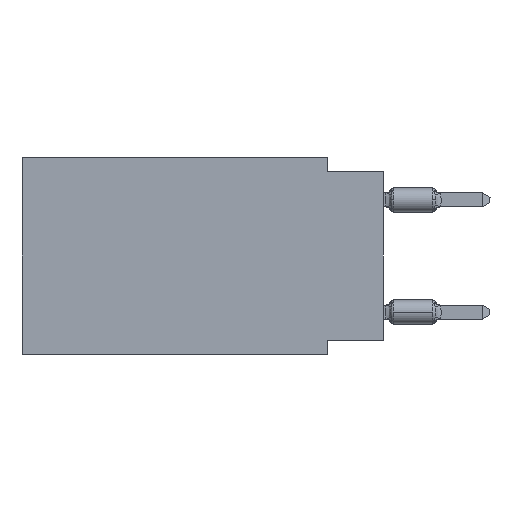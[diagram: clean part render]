
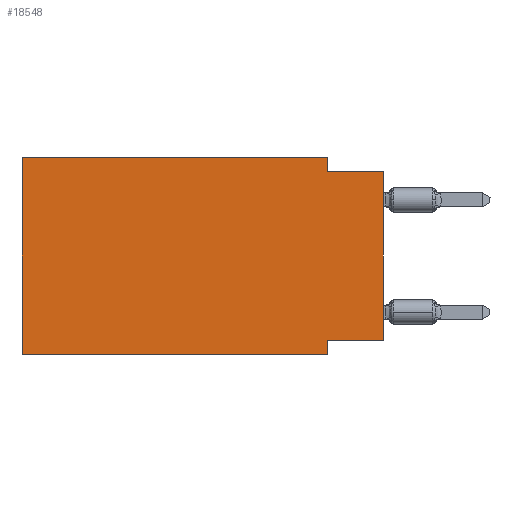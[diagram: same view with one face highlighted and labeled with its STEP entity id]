
A CAD part, left-side view. The second image highlights one B-rep face of the part: STEP entity #18548.
In plain terms, the highlighted planar face has unit normal (-1, 0, 0).
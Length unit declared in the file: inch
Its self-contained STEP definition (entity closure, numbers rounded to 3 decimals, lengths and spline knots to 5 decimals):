
#252 = CARTESIAN_POINT ( 'NONE',  ( 0., 0., -0.025 ) ) ;
#454 = LINE ( 'NONE', #33870, #2129 ) ;
#519 = CARTESIAN_POINT ( 'NONE',  ( 0., 0., -0.325 ) ) ;
#626 = ORIENTED_EDGE ( 'NONE', *, *, #19045, .F. ) ;
#1128 = LINE ( 'NONE', #47076, #40681 ) ;
#1806 = VECTOR ( 'NONE', #15934, 39.37008 ) ;
#1835 = CARTESIAN_POINT ( 'NONE',  ( 0., 0.645, 0. ) ) ;
#2129 = VECTOR ( 'NONE', #38050, 39.37008 ) ;
#2286 = ORIENTED_EDGE ( 'NONE', *, *, #26603, .F. ) ;
#3595 = VERTEX_POINT ( 'NONE', #32886 ) ;
#6285 = DIRECTION ( 'NONE',  ( 0., 0., -1. ) ) ;
#6286 = EDGE_CURVE ( 'NONE', #3595, #13347, #45619, .T. ) ;
#8643 = CARTESIAN_POINT ( 'NONE',  ( 0., 0.1, -0.35 ) ) ;
#9336 = VERTEX_POINT ( 'NONE', #29735 ) ;
#9611 = ORIENTED_EDGE ( 'NONE', *, *, #6286, .F. ) ;
#9834 = LINE ( 'NONE', #40661, #14704 ) ;
#10655 = CARTESIAN_POINT ( 'NONE',  ( 0., 0.645, -0.35 ) ) ;
#11933 = CARTESIAN_POINT ( 'NONE',  ( 0., 0.645, 0. ) ) ;
#13347 = VERTEX_POINT ( 'NONE', #52695 ) ;
#13791 = VECTOR ( 'NONE', #51740, 39.37008 ) ;
#14704 = VECTOR ( 'NONE', #43272, 39.37008 ) ;
#15934 = DIRECTION ( 'NONE',  ( 0., 1., 0. ) ) ;
#17565 = CARTESIAN_POINT ( 'NONE',  ( 0., 0.1, -0.325 ) ) ;
#17796 = EDGE_CURVE ( 'NONE', #38536, #37431, #9834, .T. ) ;
#18548 = ADVANCED_FACE ( 'NONE', ( #51949 ), #39707, .F. ) ;
#19045 = EDGE_CURVE ( 'NONE', #45640, #37431, #23745, .T. ) ;
#22667 = ORIENTED_EDGE ( 'NONE', *, *, #40851, .F. ) ;
#23195 = DIRECTION ( 'NONE',  ( 0., 0., -1. ) ) ;
#23741 = LINE ( 'NONE', #44345, #44423 ) ;
#23745 = LINE ( 'NONE', #49072, #44279 ) ;
#23896 = VERTEX_POINT ( 'NONE', #519 ) ;
#26603 = EDGE_CURVE ( 'NONE', #13347, #9336, #23741, .T. ) ;
#27650 = LINE ( 'NONE', #49610, #1806 ) ;
#29469 = DIRECTION ( 'NONE',  ( 0., -1., 0. ) ) ;
#29735 = CARTESIAN_POINT ( 'NONE',  ( 0., 0.1, -0.025 ) ) ;
#32886 = CARTESIAN_POINT ( 'NONE',  ( 0., 0.645, 0. ) ) ;
#33870 = CARTESIAN_POINT ( 'NONE',  ( 0., 0.645, 0. ) ) ;
#34836 = DIRECTION ( 'NONE',  ( 0., 0., 1. ) ) ;
#35048 = LINE ( 'NONE', #43665, #13791 ) ;
#35723 = ORIENTED_EDGE ( 'NONE', *, *, #45547, .T. ) ;
#36560 = DIRECTION ( 'NONE',  ( 0., 0., -1. ) ) ;
#37431 = VERTEX_POINT ( 'NONE', #8643 ) ;
#38050 = DIRECTION ( 'NONE',  ( 0., 0., 1. ) ) ;
#38536 = VERTEX_POINT ( 'NONE', #10655 ) ;
#39707 = PLANE ( 'NONE',  #41534 ) ;
#39979 = EDGE_CURVE ( 'NONE', #38536, #3595, #454, .T. ) ;
#40260 = DIRECTION ( 'NONE',  ( 1., 0., 0. ) ) ;
#40661 = CARTESIAN_POINT ( 'NONE',  ( 0., 0.645, -0.35 ) ) ;
#40681 = VECTOR ( 'NONE', #34836, 39.37008 ) ;
#40851 = EDGE_CURVE ( 'NONE', #9336, #40951, #35048, .T. ) ;
#40951 = VERTEX_POINT ( 'NONE', #252 ) ;
#41439 = VECTOR ( 'NONE', #29469, 39.37008 ) ;
#41534 = AXIS2_PLACEMENT_3D ( 'NONE', #1835, #40260, #6285 ) ;
#42869 = ORIENTED_EDGE ( 'NONE', *, *, #50392, .F. ) ;
#43272 = DIRECTION ( 'NONE',  ( 0., -1., 0. ) ) ;
#43665 = CARTESIAN_POINT ( 'NONE',  ( 0., 0., -0.025 ) ) ;
#43830 = EDGE_LOOP ( 'NONE', ( #35723, #22667, #2286, #9611, #51838, #49967, #626, #42869 ) ) ;
#44279 = VECTOR ( 'NONE', #36560, 39.37008 ) ;
#44345 = CARTESIAN_POINT ( 'NONE',  ( 0., 0.1, 0. ) ) ;
#44423 = VECTOR ( 'NONE', #23195, 39.37008 ) ;
#45547 = EDGE_CURVE ( 'NONE', #23896, #40951, #1128, .T. ) ;
#45619 = LINE ( 'NONE', #11933, #41439 ) ;
#45640 = VERTEX_POINT ( 'NONE', #17565 ) ;
#47076 = CARTESIAN_POINT ( 'NONE',  ( 0., 0., 0. ) ) ;
#49072 = CARTESIAN_POINT ( 'NONE',  ( 0., 0.1, -0.35 ) ) ;
#49610 = CARTESIAN_POINT ( 'NONE',  ( 0., 0., -0.325 ) ) ;
#49967 = ORIENTED_EDGE ( 'NONE', *, *, #17796, .T. ) ;
#50392 = EDGE_CURVE ( 'NONE', #23896, #45640, #27650, .T. ) ;
#51740 = DIRECTION ( 'NONE',  ( 0., -1., 0. ) ) ;
#51838 = ORIENTED_EDGE ( 'NONE', *, *, #39979, .F. ) ;
#51949 = FACE_OUTER_BOUND ( 'NONE', #43830, .T. ) ;
#52695 = CARTESIAN_POINT ( 'NONE',  ( 0., 0.1, 0. ) ) ;
